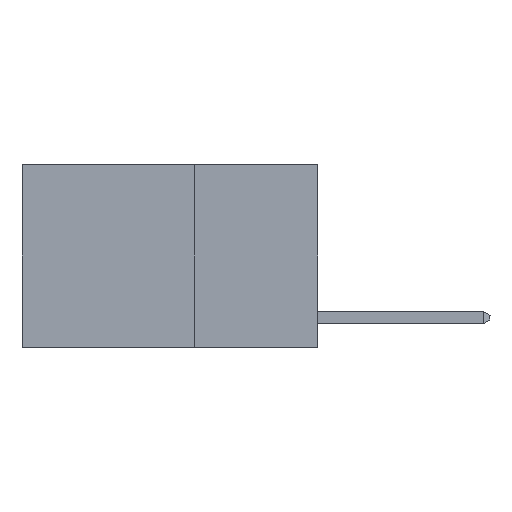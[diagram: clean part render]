
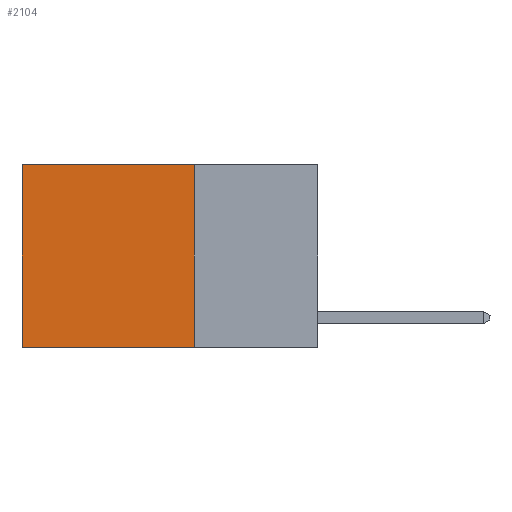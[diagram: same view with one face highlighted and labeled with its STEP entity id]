
A CAD part, left-side view. The second image highlights one B-rep face of the part: STEP entity #2104.
In plain terms, the highlighted planar face has unit normal (-1, 0, 0).
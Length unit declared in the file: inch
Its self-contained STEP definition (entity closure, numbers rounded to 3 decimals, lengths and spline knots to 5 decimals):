
#1096 = AXIS2_PLACEMENT_3D ( 'NONE', #2758, #11755, #8394 ) ;
#1592 = ORIENTED_EDGE ( 'NONE', *, *, #4628, .T. ) ;
#1891 = VECTOR ( 'NONE', #11049, 39.37008 ) ;
#1949 = CARTESIAN_POINT ( 'NONE',  ( 0.2625, 0.25, 0. ) ) ;
#2104 = ADVANCED_FACE ( 'NONE', ( #10777 ), #16388, .F. ) ;
#2372 = LINE ( 'NONE', #14890, #10037 ) ;
#2535 = VECTOR ( 'NONE', #18239, 39.37008 ) ;
#2758 = CARTESIAN_POINT ( 'NONE',  ( 0.2625, 0.25, 0. ) ) ;
#3070 = DIRECTION ( 'NONE',  ( 0., 0., -1. ) ) ;
#4551 = VERTEX_POINT ( 'NONE', #16307 ) ;
#4555 = VERTEX_POINT ( 'NONE', #12172 ) ;
#4628 = EDGE_CURVE ( 'NONE', #13249, #8089, #13997, .T. ) ;
#5277 = ORIENTED_EDGE ( 'NONE', *, *, #10599, .T. ) ;
#8089 = VERTEX_POINT ( 'NONE', #12839 ) ;
#8394 = DIRECTION ( 'NONE',  ( 0., 0., -1. ) ) ;
#9289 = DIRECTION ( 'NONE',  ( 0., 1., 0. ) ) ;
#9630 = VECTOR ( 'NONE', #3070, 39.37008 ) ;
#10037 = VECTOR ( 'NONE', #9289, 39.37008 ) ;
#10599 = EDGE_CURVE ( 'NONE', #8089, #4555, #11359, .T. ) ;
#10777 = FACE_OUTER_BOUND ( 'NONE', #12427, .T. ) ;
#11049 = DIRECTION ( 'NONE',  ( 0., 1., 0. ) ) ;
#11241 = CARTESIAN_POINT ( 'NONE',  ( 0.2625, 0.25, 0. ) ) ;
#11348 = EDGE_CURVE ( 'NONE', #13249, #4551, #12595, .T. ) ;
#11359 = LINE ( 'NONE', #14391, #9630 ) ;
#11755 = DIRECTION ( 'NONE',  ( 1., 0., 0. ) ) ;
#12172 = CARTESIAN_POINT ( 'NONE',  ( 0.2625, 0.6, -0.37 ) ) ;
#12427 = EDGE_LOOP ( 'NONE', ( #5277, #12787, #13807, #1592 ) ) ;
#12595 = LINE ( 'NONE', #15620, #2535 ) ;
#12787 = ORIENTED_EDGE ( 'NONE', *, *, #16047, .F. ) ;
#12839 = CARTESIAN_POINT ( 'NONE',  ( 0.2625, 0.6, 0. ) ) ;
#13249 = VERTEX_POINT ( 'NONE', #1949 ) ;
#13807 = ORIENTED_EDGE ( 'NONE', *, *, #11348, .F. ) ;
#13997 = LINE ( 'NONE', #11241, #1891 ) ;
#14391 = CARTESIAN_POINT ( 'NONE',  ( 0.2625, 0.6, 0. ) ) ;
#14890 = CARTESIAN_POINT ( 'NONE',  ( 0.2625, 0.25, -0.37 ) ) ;
#15620 = CARTESIAN_POINT ( 'NONE',  ( 0.2625, 0.25, 0. ) ) ;
#16047 = EDGE_CURVE ( 'NONE', #4551, #4555, #2372, .T. ) ;
#16307 = CARTESIAN_POINT ( 'NONE',  ( 0.2625, 0.25, -0.37 ) ) ;
#16388 = PLANE ( 'NONE',  #1096 ) ;
#18239 = DIRECTION ( 'NONE',  ( 0., 0., -1. ) ) ;
